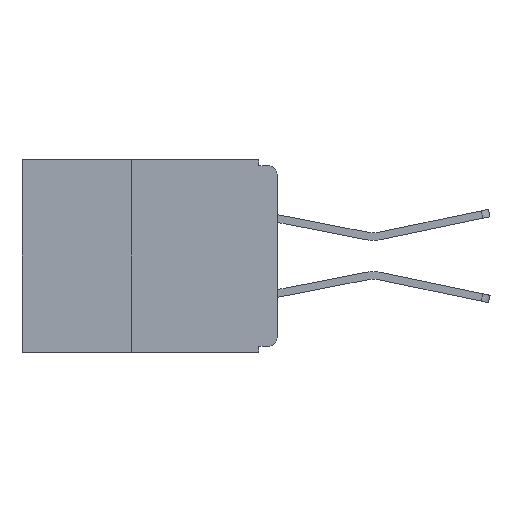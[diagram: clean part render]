
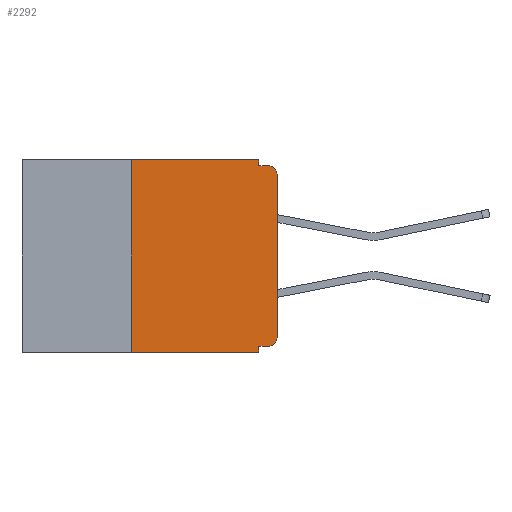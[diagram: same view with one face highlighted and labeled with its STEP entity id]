
A CAD part, left-side view. The second image highlights one B-rep face of the part: STEP entity #2292.
In plain terms, the highlighted planar face has unit normal (-1, 0, 0).
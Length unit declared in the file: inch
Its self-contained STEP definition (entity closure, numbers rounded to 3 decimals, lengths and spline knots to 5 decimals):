
#92 = CARTESIAN_POINT ( 'NONE',  ( 0., 0.031, -0.01 ) ) ;
#365 = LINE ( 'NONE', #15278, #4123 ) ;
#618 = CARTESIAN_POINT ( 'NONE',  ( 0., 0.437, 0. ) ) ;
#1286 = EDGE_CURVE ( 'NONE', #14520, #11493, #15413, .T. ) ;
#1305 = DIRECTION ( 'NONE',  ( -1., 0., 0. ) ) ;
#1400 = VERTEX_POINT ( 'NONE', #92 ) ;
#1411 = EDGE_CURVE ( 'NONE', #5741, #1400, #16842, .T. ) ;
#1423 = CARTESIAN_POINT ( 'NONE',  ( 0., 0.015, -0.025 ) ) ;
#1870 = EDGE_CURVE ( 'NONE', #4277, #17309, #14149, .T. ) ;
#2292 = ADVANCED_FACE ( 'NONE', ( #10528 ), #15945, .F. ) ;
#2329 = VERTEX_POINT ( 'NONE', #11956 ) ;
#2346 = VECTOR ( 'NONE', #15120, 39.37008 ) ;
#3679 = LINE ( 'NONE', #16514, #6902 ) ;
#3772 = ORIENTED_EDGE ( 'NONE', *, *, #15108, .F. ) ;
#3817 = EDGE_CURVE ( 'NONE', #17309, #14849, #5542, .T. ) ;
#4088 = VECTOR ( 'NONE', #6024, 39.37008 ) ;
#4123 = VECTOR ( 'NONE', #7144, 39.37008 ) ;
#4151 = VERTEX_POINT ( 'NONE', #10106 ) ;
#4204 = ORIENTED_EDGE ( 'NONE', *, *, #15542, .T. ) ;
#4277 = VERTEX_POINT ( 'NONE', #4890 ) ;
#4851 = DIRECTION ( 'NONE',  ( 0., -1., 0. ) ) ;
#4890 = CARTESIAN_POINT ( 'NONE',  ( 0., 0.015, -0.32 ) ) ;
#5050 = AXIS2_PLACEMENT_3D ( 'NONE', #1423, #1305, #9467 ) ;
#5164 = AXIS2_PLACEMENT_3D ( 'NONE', #6374, #15867, #7735 ) ;
#5334 = CARTESIAN_POINT ( 'NONE',  ( 0., 0.031, -0.33 ) ) ;
#5421 = CARTESIAN_POINT ( 'NONE',  ( 0., 0.015, -0.01 ) ) ;
#5448 = CARTESIAN_POINT ( 'NONE',  ( 0., 0.031, 0. ) ) ;
#5542 = LINE ( 'NONE', #5334, #12389 ) ;
#5741 = VERTEX_POINT ( 'NONE', #5448 ) ;
#5743 = CARTESIAN_POINT ( 'NONE',  ( 0., 0.031, -0.32 ) ) ;
#6024 = DIRECTION ( 'NONE',  ( 0., 0., 1. ) ) ;
#6374 = CARTESIAN_POINT ( 'NONE',  ( 0., 0.015, -0.305 ) ) ;
#6467 = LINE ( 'NONE', #16449, #2346 ) ;
#6491 = ORIENTED_EDGE ( 'NONE', *, *, #15988, .F. ) ;
#6649 = ORIENTED_EDGE ( 'NONE', *, *, #16302, .T. ) ;
#6900 = VECTOR ( 'NONE', #12288, 39.37008 ) ;
#6902 = VECTOR ( 'NONE', #15202, 39.37008 ) ;
#7039 = DIRECTION ( 'NONE',  ( 0., 0., -1. ) ) ;
#7144 = DIRECTION ( 'NONE',  ( 0., -1., 0. ) ) ;
#7405 = CARTESIAN_POINT ( 'NONE',  ( 0., 0., 0. ) ) ;
#7570 = ORIENTED_EDGE ( 'NONE', *, *, #3817, .F. ) ;
#7735 = DIRECTION ( 'NONE',  ( 0., 0., -1. ) ) ;
#9186 = ORIENTED_EDGE ( 'NONE', *, *, #14426, .F. ) ;
#9229 = EDGE_CURVE ( 'NONE', #2329, #14520, #14962, .T. ) ;
#9467 = DIRECTION ( 'NONE',  ( 0., 0., -1. ) ) ;
#9796 = CARTESIAN_POINT ( 'NONE',  ( 0., 0.25, -0.33 ) ) ;
#9993 = CARTESIAN_POINT ( 'NONE',  ( 0., 0.031, 0. ) ) ;
#10071 = CARTESIAN_POINT ( 'NONE',  ( 0., 0., -0.025 ) ) ;
#10106 = CARTESIAN_POINT ( 'NONE',  ( 0., 0.25, 0. ) ) ;
#10133 = VECTOR ( 'NONE', #4851, 39.37008 ) ;
#10528 = FACE_OUTER_BOUND ( 'NONE', #14734, .T. ) ;
#11040 = DIRECTION ( 'NONE',  ( 0., 0., -1. ) ) ;
#11111 = DIRECTION ( 'NONE',  ( 1., 0., 0. ) ) ;
#11360 = AXIS2_PLACEMENT_3D ( 'NONE', #15600, #11111, #11040 ) ;
#11364 = CIRCLE ( 'NONE', #5164, 0.015 ) ;
#11493 = VERTEX_POINT ( 'NONE', #5421 ) ;
#11956 = CARTESIAN_POINT ( 'NONE',  ( 0., 0., -0.305 ) ) ;
#12239 = ORIENTED_EDGE ( 'NONE', *, *, #9229, .T. ) ;
#12288 = DIRECTION ( 'NONE',  ( 0., 1., 0. ) ) ;
#12389 = VECTOR ( 'NONE', #13512, 39.37008 ) ;
#12402 = CARTESIAN_POINT ( 'NONE',  ( 0., 0.031, -0.33 ) ) ;
#12425 = ORIENTED_EDGE ( 'NONE', *, *, #1286, .T. ) ;
#13335 = VECTOR ( 'NONE', #7039, 39.37008 ) ;
#13512 = DIRECTION ( 'NONE',  ( 0., 0., -1. ) ) ;
#13752 = LINE ( 'NONE', #618, #10133 ) ;
#13788 = VERTEX_POINT ( 'NONE', #9796 ) ;
#14149 = LINE ( 'NONE', #15122, #6900 ) ;
#14426 = EDGE_CURVE ( 'NONE', #1400, #11493, #365, .T. ) ;
#14520 = VERTEX_POINT ( 'NONE', #10071 ) ;
#14734 = EDGE_LOOP ( 'NONE', ( #12239, #12425, #9186, #16063, #3772, #6491, #4204, #7570, #15873, #6649 ) ) ;
#14849 = VERTEX_POINT ( 'NONE', #12402 ) ;
#14962 = LINE ( 'NONE', #7405, #4088 ) ;
#15108 = EDGE_CURVE ( 'NONE', #4151, #5741, #13752, .T. ) ;
#15120 = DIRECTION ( 'NONE',  ( 0., 0., 1. ) ) ;
#15122 = CARTESIAN_POINT ( 'NONE',  ( 0., 0., -0.32 ) ) ;
#15202 = DIRECTION ( 'NONE',  ( 0., -1., 0. ) ) ;
#15278 = CARTESIAN_POINT ( 'NONE',  ( 0., 0., -0.01 ) ) ;
#15413 = CIRCLE ( 'NONE', #5050, 0.015 ) ;
#15542 = EDGE_CURVE ( 'NONE', #13788, #14849, #3679, .T. ) ;
#15600 = CARTESIAN_POINT ( 'NONE',  ( 0., 0.437, 0. ) ) ;
#15867 = DIRECTION ( 'NONE',  ( -1., 0., 0. ) ) ;
#15873 = ORIENTED_EDGE ( 'NONE', *, *, #1870, .F. ) ;
#15945 = PLANE ( 'NONE',  #11360 ) ;
#15988 = EDGE_CURVE ( 'NONE', #13788, #4151, #6467, .T. ) ;
#16063 = ORIENTED_EDGE ( 'NONE', *, *, #1411, .F. ) ;
#16302 = EDGE_CURVE ( 'NONE', #4277, #2329, #11364, .T. ) ;
#16449 = CARTESIAN_POINT ( 'NONE',  ( 0., 0.25, -0.33 ) ) ;
#16514 = CARTESIAN_POINT ( 'NONE',  ( 0., 0.437, -0.33 ) ) ;
#16842 = LINE ( 'NONE', #9993, #13335 ) ;
#17309 = VERTEX_POINT ( 'NONE', #5743 ) ;
